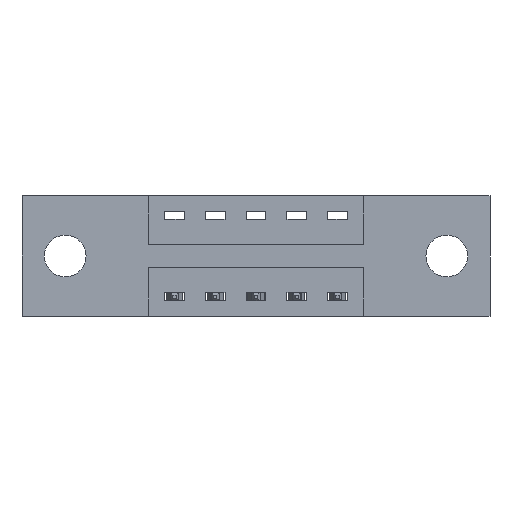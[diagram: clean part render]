
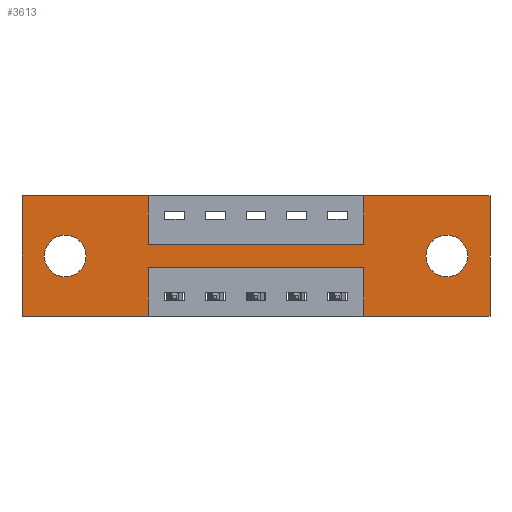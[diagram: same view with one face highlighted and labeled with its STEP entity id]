
A CAD part, front view. The second image highlights one B-rep face of the part: STEP entity #3613.
In plain terms, the highlighted planar face has unit normal (0, -1, 0).
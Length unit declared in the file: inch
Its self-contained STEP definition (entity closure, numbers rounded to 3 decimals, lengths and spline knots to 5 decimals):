
#120 = ORIENTED_EDGE ( 'NONE', *, *, #2962, .F. ) ;
#130 = DIRECTION ( 'NONE',  ( 0., 1., 0. ) ) ;
#237 = ORIENTED_EDGE ( 'NONE', *, *, #320, .T. ) ;
#280 = VERTEX_POINT ( 'NONE', #2722 ) ;
#320 = EDGE_CURVE ( 'NONE', #7270, #4898, #2946, .T. ) ;
#360 = CARTESIAN_POINT ( 'NONE',  ( 0.3875, 0., -0.37 ) ) ;
#418 = VERTEX_POINT ( 'NONE', #3478 ) ;
#461 = ORIENTED_EDGE ( 'NONE', *, *, #7806, .F. ) ;
#593 = VECTOR ( 'NONE', #7231, 39.37008 ) ;
#647 = CARTESIAN_POINT ( 'NONE',  ( 0., 0., -0.37 ) ) ;
#681 = AXIS2_PLACEMENT_3D ( 'NONE', #3927, #130, #4553 ) ;
#713 = AXIS2_PLACEMENT_3D ( 'NONE', #4662, #864, #5294 ) ;
#827 = LINE ( 'NONE', #647, #7287 ) ;
#864 = DIRECTION ( 'NONE',  ( 0., 1., 0. ) ) ;
#883 = VECTOR ( 'NONE', #5063, 39.37008 ) ;
#902 = DIRECTION ( 'NONE',  ( 0., 0., -1. ) ) ;
#1081 = CARTESIAN_POINT ( 'NONE',  ( 0., 0., -0.37 ) ) ;
#1085 = CARTESIAN_POINT ( 'NONE',  ( 0.3875, 0., -0.37 ) ) ;
#1101 = CARTESIAN_POINT ( 'NONE',  ( 0., 0., 0. ) ) ;
#1165 = CARTESIAN_POINT ( 'NONE',  ( 0., 0., 0. ) ) ;
#1188 = VERTEX_POINT ( 'NONE', #8098 ) ;
#1231 = LINE ( 'NONE', #5802, #4389 ) ;
#1241 = VECTOR ( 'NONE', #902, 39.37008 ) ;
#1346 = EDGE_CURVE ( 'NONE', #1188, #5827, #5686, .T. ) ;
#1452 = EDGE_CURVE ( 'NONE', #280, #1880, #6170, .T. ) ;
#1520 = VECTOR ( 'NONE', #2052, 39.37008 ) ;
#1521 = LINE ( 'NONE', #2554, #3206 ) ;
#1546 = ORIENTED_EDGE ( 'NONE', *, *, #7669, .F. ) ;
#1559 = CARTESIAN_POINT ( 'NONE',  ( 1.3025, 0., -0.185 ) ) ;
#1572 = VERTEX_POINT ( 'NONE', #7196 ) ;
#1729 = VECTOR ( 'NONE', #6281, 39.37008 ) ;
#1880 = VERTEX_POINT ( 'NONE', #5153 ) ;
#2047 = DIRECTION ( 'NONE',  ( -1., 0., 0. ) ) ;
#2052 = DIRECTION ( 'NONE',  ( 0., 0., -1. ) ) ;
#2057 = CARTESIAN_POINT ( 'NONE',  ( 1.435, 0., 0. ) ) ;
#2081 = EDGE_CURVE ( 'NONE', #4898, #7270, #3306, .T. ) ;
#2089 = CARTESIAN_POINT ( 'NONE',  ( 1.0475, 0., 0. ) ) ;
#2092 = ORIENTED_EDGE ( 'NONE', *, *, #1452, .F. ) ;
#2151 = AXIS2_PLACEMENT_3D ( 'NONE', #6525, #2767, #7133 ) ;
#2197 = DIRECTION ( 'NONE',  ( 0., 0., -1. ) ) ;
#2270 = LINE ( 'NONE', #360, #593 ) ;
#2297 = CARTESIAN_POINT ( 'NONE',  ( 1.435, 0., -0.37 ) ) ;
#2340 = EDGE_CURVE ( 'NONE', #5489, #280, #1521, .T. ) ;
#2356 = PLANE ( 'NONE',  #4716 ) ;
#2475 = EDGE_CURVE ( 'NONE', #5230, #7738, #5368, .T. ) ;
#2496 = ORIENTED_EDGE ( 'NONE', *, *, #5636, .F. ) ;
#2505 = CIRCLE ( 'NONE', #713, 0.064 ) ;
#2554 = CARTESIAN_POINT ( 'NONE',  ( 0., 0., -0.37 ) ) ;
#2597 = ORIENTED_EDGE ( 'NONE', *, *, #2475, .F. ) ;
#2680 = ORIENTED_EDGE ( 'NONE', *, *, #4565, .T. ) ;
#2717 = FACE_OUTER_BOUND ( 'NONE', #5812, .T. ) ;
#2722 = CARTESIAN_POINT ( 'NONE',  ( 0., 0., -0.37 ) ) ;
#2767 = DIRECTION ( 'NONE',  ( 0., 1., 0. ) ) ;
#2789 = CARTESIAN_POINT ( 'NONE',  ( 0.3875, 0., 0. ) ) ;
#2797 = CARTESIAN_POINT ( 'NONE',  ( 0.1325, 0., -0.121 ) ) ;
#2800 = LINE ( 'NONE', #1165, #7764 ) ;
#2946 = CIRCLE ( 'NONE', #2151, 0.064 ) ;
#2962 = EDGE_CURVE ( 'NONE', #7738, #5676, #7293, .T. ) ;
#3087 = ORIENTED_EDGE ( 'NONE', *, *, #4301, .F. ) ;
#3202 = LINE ( 'NONE', #6441, #1520 ) ;
#3206 = VECTOR ( 'NONE', #6932, 39.37008 ) ;
#3234 = CARTESIAN_POINT ( 'NONE',  ( 1.0475, 0., 0. ) ) ;
#3306 = CIRCLE ( 'NONE', #5020, 0.064 ) ;
#3478 = CARTESIAN_POINT ( 'NONE',  ( 0.3875, 0., 0. ) ) ;
#3553 = VERTEX_POINT ( 'NONE', #2297 ) ;
#3613 = ADVANCED_FACE ( 'NONE', ( #7683, #6069, #2717 ), #2356, .T. ) ;
#3622 = DIRECTION ( 'NONE',  ( 0., -1., 0. ) ) ;
#3695 = CARTESIAN_POINT ( 'NONE',  ( 1.3025, 0., -0.249 ) ) ;
#3927 = CARTESIAN_POINT ( 'NONE',  ( 0.1325, 0., -0.185 ) ) ;
#3985 = ORIENTED_EDGE ( 'NONE', *, *, #2340, .F. ) ;
#4013 = CARTESIAN_POINT ( 'NONE',  ( 0., 0., 0. ) ) ;
#4038 = EDGE_CURVE ( 'NONE', #418, #7026, #4591, .T. ) ;
#4074 = ORIENTED_EDGE ( 'NONE', *, *, #4500, .F. ) ;
#4160 = VERTEX_POINT ( 'NONE', #6666 ) ;
#4301 = EDGE_CURVE ( 'NONE', #1880, #418, #2800, .T. ) ;
#4389 = VECTOR ( 'NONE', #2047, 39.37008 ) ;
#4472 = ORIENTED_EDGE ( 'NONE', *, *, #5190, .F. ) ;
#4500 = EDGE_CURVE ( 'NONE', #5839, #1572, #1231, .T. ) ;
#4518 = VECTOR ( 'NONE', #7707, 39.37008 ) ;
#4553 = DIRECTION ( 'NONE',  ( 0., 0., 1. ) ) ;
#4565 = EDGE_CURVE ( 'NONE', #5827, #1188, #2505, .T. ) ;
#4591 = LINE ( 'NONE', #2789, #1241 ) ;
#4662 = CARTESIAN_POINT ( 'NONE',  ( 0.1325, 0., -0.185 ) ) ;
#4712 = CARTESIAN_POINT ( 'NONE',  ( 1.3025, 0., -0.121 ) ) ;
#4716 = AXIS2_PLACEMENT_3D ( 'NONE', #1081, #3622, #7970 ) ;
#4741 = CARTESIAN_POINT ( 'NONE',  ( 0.3875, 0., -0.15 ) ) ;
#4898 = VERTEX_POINT ( 'NONE', #3695 ) ;
#5020 = AXIS2_PLACEMENT_3D ( 'NONE', #1559, #5977, #2197 ) ;
#5063 = DIRECTION ( 'NONE',  ( 1., 0., 0. ) ) ;
#5153 = CARTESIAN_POINT ( 'NONE',  ( 0., 0., 0. ) ) ;
#5190 = EDGE_CURVE ( 'NONE', #4160, #5839, #7367, .T. ) ;
#5230 = VERTEX_POINT ( 'NONE', #6529 ) ;
#5294 = DIRECTION ( 'NONE',  ( 0., 0., 1. ) ) ;
#5368 = LINE ( 'NONE', #2089, #7576 ) ;
#5489 = VERTEX_POINT ( 'NONE', #1085 ) ;
#5576 = DIRECTION ( 'NONE',  ( 1., 0., 0. ) ) ;
#5620 = CARTESIAN_POINT ( 'NONE',  ( 0.3875, 0., -0.15 ) ) ;
#5636 = EDGE_CURVE ( 'NONE', #7026, #5230, #7545, .T. ) ;
#5676 = VERTEX_POINT ( 'NONE', #2057 ) ;
#5686 = CIRCLE ( 'NONE', #681, 0.064 ) ;
#5734 = VECTOR ( 'NONE', #7116, 39.37008 ) ;
#5746 = ORIENTED_EDGE ( 'NONE', *, *, #4038, .F. ) ;
#5802 = CARTESIAN_POINT ( 'NONE',  ( 0.3875, 0., -0.22 ) ) ;
#5812 = EDGE_LOOP ( 'NONE', ( #7715, #4074, #4472, #1546, #461, #120, #2597, #2496, #5746, #3087, #2092, #3985 ) ) ;
#5827 = VERTEX_POINT ( 'NONE', #2797 ) ;
#5839 = VERTEX_POINT ( 'NONE', #5961 ) ;
#5907 = EDGE_CURVE ( 'NONE', #1572, #5489, #2270, .T. ) ;
#5961 = CARTESIAN_POINT ( 'NONE',  ( 1.0475, 0., -0.22 ) ) ;
#5977 = DIRECTION ( 'NONE',  ( 0., 1., 0. ) ) ;
#6069 = FACE_BOUND ( 'NONE', #6701, .T. ) ;
#6170 = LINE ( 'NONE', #4013, #4518 ) ;
#6281 = DIRECTION ( 'NONE',  ( 1., 0., 0. ) ) ;
#6283 = ORIENTED_EDGE ( 'NONE', *, *, #1346, .T. ) ;
#6441 = CARTESIAN_POINT ( 'NONE',  ( 1.435, 0., 0. ) ) ;
#6473 = DIRECTION ( 'NONE',  ( 0., 0., 1. ) ) ;
#6497 = CARTESIAN_POINT ( 'NONE',  ( 1.0475, 0., -0.37 ) ) ;
#6525 = CARTESIAN_POINT ( 'NONE',  ( 1.3025, 0., -0.185 ) ) ;
#6529 = CARTESIAN_POINT ( 'NONE',  ( 1.0475, 0., -0.15 ) ) ;
#6666 = CARTESIAN_POINT ( 'NONE',  ( 1.0475, 0., -0.37 ) ) ;
#6701 = EDGE_LOOP ( 'NONE', ( #2680, #6283 ) ) ;
#6932 = DIRECTION ( 'NONE',  ( -1., 0., 0. ) ) ;
#7026 = VERTEX_POINT ( 'NONE', #5620 ) ;
#7116 = DIRECTION ( 'NONE',  ( 0., 0., 1. ) ) ;
#7133 = DIRECTION ( 'NONE',  ( 0., 0., -1. ) ) ;
#7196 = CARTESIAN_POINT ( 'NONE',  ( 0.3875, 0., -0.22 ) ) ;
#7231 = DIRECTION ( 'NONE',  ( 0., 0., -1. ) ) ;
#7270 = VERTEX_POINT ( 'NONE', #4712 ) ;
#7287 = VECTOR ( 'NONE', #7525, 39.37008 ) ;
#7293 = LINE ( 'NONE', #1101, #1729 ) ;
#7367 = LINE ( 'NONE', #6497, #5734 ) ;
#7525 = DIRECTION ( 'NONE',  ( -1., 0., 0. ) ) ;
#7545 = LINE ( 'NONE', #4741, #883 ) ;
#7576 = VECTOR ( 'NONE', #6473, 39.37008 ) ;
#7669 = EDGE_CURVE ( 'NONE', #3553, #4160, #827, .T. ) ;
#7683 = FACE_BOUND ( 'NONE', #7835, .T. ) ;
#7707 = DIRECTION ( 'NONE',  ( 0., 0., 1. ) ) ;
#7715 = ORIENTED_EDGE ( 'NONE', *, *, #5907, .F. ) ;
#7738 = VERTEX_POINT ( 'NONE', #3234 ) ;
#7764 = VECTOR ( 'NONE', #5576, 39.37008 ) ;
#7806 = EDGE_CURVE ( 'NONE', #5676, #3553, #3202, .T. ) ;
#7835 = EDGE_LOOP ( 'NONE', ( #237, #7982 ) ) ;
#7970 = DIRECTION ( 'NONE',  ( 0., 0., -1. ) ) ;
#7982 = ORIENTED_EDGE ( 'NONE', *, *, #2081, .T. ) ;
#8098 = CARTESIAN_POINT ( 'NONE',  ( 0.1325, 0., -0.249 ) ) ;
